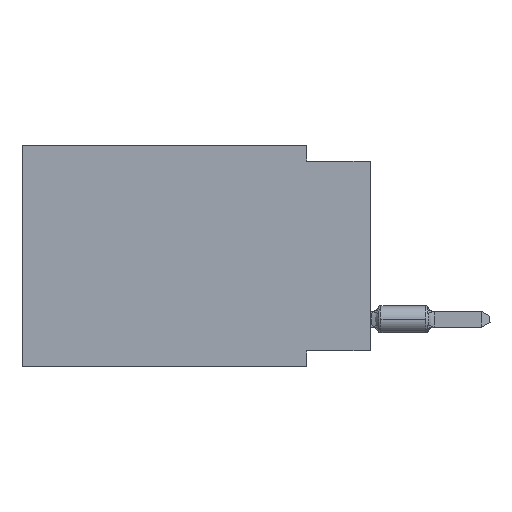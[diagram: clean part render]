
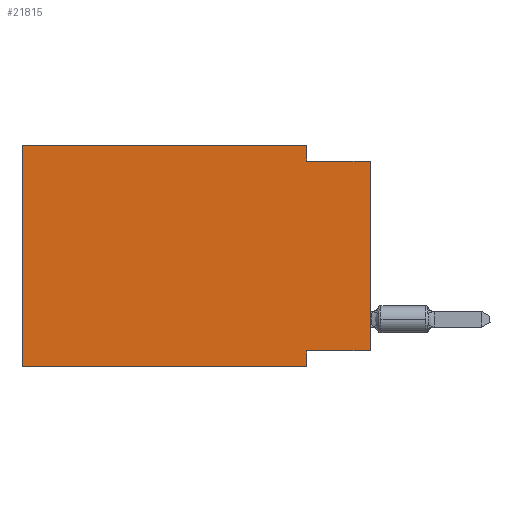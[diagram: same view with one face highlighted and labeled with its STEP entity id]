
A CAD part, left-side view. The second image highlights one B-rep face of the part: STEP entity #21815.
In plain terms, the highlighted planar face has unit normal (-1, 0, 0).
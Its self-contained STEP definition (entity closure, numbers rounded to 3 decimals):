
#2795 = DIRECTION ( 'NONE',  ( 0., 0., 1. ) ) ;
#3506 = VECTOR ( 'NONE', #48975, 1000. ) ;
#3899 = LINE ( 'NONE', #33461, #44120 ) ;
#4220 = CARTESIAN_POINT ( 'NONE',  ( 0., 0., -0.635 ) ) ;
#4609 = CARTESIAN_POINT ( 'NONE',  ( 0., 13.97, 0. ) ) ;
#5089 = CARTESIAN_POINT ( 'NONE',  ( 0., 13.97, -8.89 ) ) ;
#5862 = VERTEX_POINT ( 'NONE', #46007 ) ;
#6994 = VERTEX_POINT ( 'NONE', #33050 ) ;
#7346 = FACE_OUTER_BOUND ( 'NONE', #27759, .T. ) ;
#7974 = DIRECTION ( 'NONE',  ( 0., 0., 1. ) ) ;
#8133 = VERTEX_POINT ( 'NONE', #50544 ) ;
#10547 = CARTESIAN_POINT ( 'NONE',  ( 0., 2.54, -8.89 ) ) ;
#10705 = ORIENTED_EDGE ( 'NONE', *, *, #33035, .T. ) ;
#12237 = DIRECTION ( 'NONE',  ( 0., 0., -1. ) ) ;
#13295 = VECTOR ( 'NONE', #38487, 1000. ) ;
#13524 = LINE ( 'NONE', #5089, #44016 ) ;
#13655 = VERTEX_POINT ( 'NONE', #28711 ) ;
#13935 = EDGE_CURVE ( 'NONE', #6994, #35618, #48857, .T. ) ;
#14138 = ORIENTED_EDGE ( 'NONE', *, *, #18957, .F. ) ;
#14221 = VECTOR ( 'NONE', #24572, 1000. ) ;
#15150 = VECTOR ( 'NONE', #2795, 1000. ) ;
#15775 = PLANE ( 'NONE',  #29668 ) ;
#16439 = CARTESIAN_POINT ( 'NONE',  ( 0., 13.97, 0. ) ) ;
#16813 = LINE ( 'NONE', #37127, #15150 ) ;
#16837 = DIRECTION ( 'NONE',  ( 1., 0., 0. ) ) ;
#18696 = DIRECTION ( 'NONE',  ( 0., 0., -1. ) ) ;
#18957 = EDGE_CURVE ( 'NONE', #35618, #13655, #24324, .T. ) ;
#20463 = CARTESIAN_POINT ( 'NONE',  ( 0., 13.97, -8.89 ) ) ;
#20697 = ORIENTED_EDGE ( 'NONE', *, *, #26071, .F. ) ;
#21815 = ADVANCED_FACE ( 'NONE', ( #7346 ), #15775, .F. ) ;
#21953 = LINE ( 'NONE', #22495, #13295 ) ;
#22495 = CARTESIAN_POINT ( 'NONE',  ( 0., 0., -8.255 ) ) ;
#22676 = CARTESIAN_POINT ( 'NONE',  ( 0., 0., -8.255 ) ) ;
#22706 = EDGE_CURVE ( 'NONE', #32214, #6994, #24847, .T. ) ;
#22851 = ORIENTED_EDGE ( 'NONE', *, *, #22706, .F. ) ;
#24324 = LINE ( 'NONE', #4220, #3506 ) ;
#24572 = DIRECTION ( 'NONE',  ( 0., -1., 0. ) ) ;
#24847 = LINE ( 'NONE', #16439, #14221 ) ;
#26071 = EDGE_CURVE ( 'NONE', #48307, #5862, #21953, .T. ) ;
#27313 = VECTOR ( 'NONE', #18696, 1000. ) ;
#27759 = EDGE_LOOP ( 'NONE', ( #10705, #14138, #52194, #22851, #52260, #41638, #41198, #20697 ) ) ;
#28711 = CARTESIAN_POINT ( 'NONE',  ( 0., 0., -0.635 ) ) ;
#29668 = AXIS2_PLACEMENT_3D ( 'NONE', #4609, #16837, #12237 ) ;
#30988 = VECTOR ( 'NONE', #40210, 1000. ) ;
#32214 = VERTEX_POINT ( 'NONE', #32457 ) ;
#32457 = CARTESIAN_POINT ( 'NONE',  ( 0., 13.97, 0. ) ) ;
#33035 = EDGE_CURVE ( 'NONE', #48307, #13655, #16813, .T. ) ;
#33050 = CARTESIAN_POINT ( 'NONE',  ( 0., 2.54, 0. ) ) ;
#33461 = CARTESIAN_POINT ( 'NONE',  ( 0., 13.97, 0. ) ) ;
#33686 = EDGE_CURVE ( 'NONE', #5862, #8133, #51227, .T. ) ;
#34653 = DIRECTION ( 'NONE',  ( 0., -1., 0. ) ) ;
#35618 = VERTEX_POINT ( 'NONE', #50675 ) ;
#37127 = CARTESIAN_POINT ( 'NONE',  ( 0., 0., 0. ) ) ;
#38487 = DIRECTION ( 'NONE',  ( 0., 1., 0. ) ) ;
#40210 = DIRECTION ( 'NONE',  ( 0., 0., -1. ) ) ;
#40441 = VERTEX_POINT ( 'NONE', #20463 ) ;
#41198 = ORIENTED_EDGE ( 'NONE', *, *, #33686, .F. ) ;
#41638 = ORIENTED_EDGE ( 'NONE', *, *, #50731, .T. ) ;
#44016 = VECTOR ( 'NONE', #34653, 1000. ) ;
#44120 = VECTOR ( 'NONE', #7974, 1000. ) ;
#46007 = CARTESIAN_POINT ( 'NONE',  ( 0., 2.54, -8.255 ) ) ;
#48307 = VERTEX_POINT ( 'NONE', #22676 ) ;
#48338 = CARTESIAN_POINT ( 'NONE',  ( 0., 2.54, 0. ) ) ;
#48546 = EDGE_CURVE ( 'NONE', #40441, #32214, #3899, .T. ) ;
#48857 = LINE ( 'NONE', #48338, #30988 ) ;
#48975 = DIRECTION ( 'NONE',  ( 0., -1., 0. ) ) ;
#50544 = CARTESIAN_POINT ( 'NONE',  ( 0., 2.54, -8.89 ) ) ;
#50675 = CARTESIAN_POINT ( 'NONE',  ( 0., 2.54, -0.635 ) ) ;
#50731 = EDGE_CURVE ( 'NONE', #40441, #8133, #13524, .T. ) ;
#51227 = LINE ( 'NONE', #10547, #27313 ) ;
#52194 = ORIENTED_EDGE ( 'NONE', *, *, #13935, .F. ) ;
#52260 = ORIENTED_EDGE ( 'NONE', *, *, #48546, .F. ) ;
